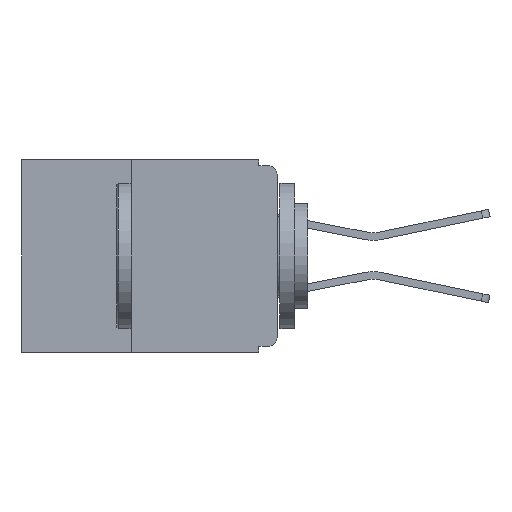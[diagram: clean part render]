
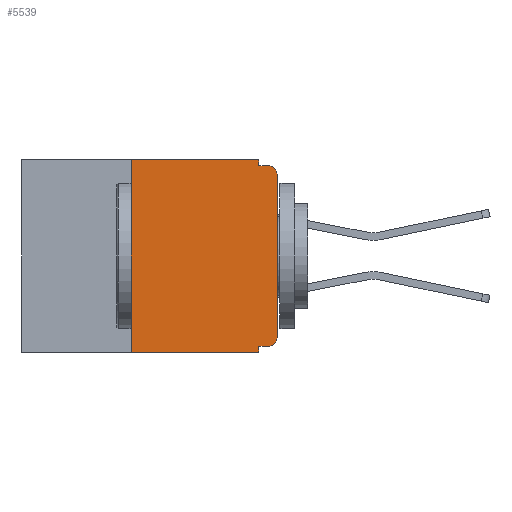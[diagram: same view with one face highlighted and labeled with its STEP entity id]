
A CAD part, left-side view. The second image highlights one B-rep face of the part: STEP entity #5539.
In plain terms, the highlighted planar face has unit normal (-1, 0, 0).
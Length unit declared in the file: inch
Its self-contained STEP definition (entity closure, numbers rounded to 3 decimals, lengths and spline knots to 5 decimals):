
#279 = CARTESIAN_POINT ( 'NONE',  ( 0., 0.031, 0. ) ) ;
#623 = EDGE_CURVE ( 'NONE', #16920, #27429, #1084, .T. ) ;
#801 = DIRECTION ( 'NONE',  ( 0., 0., 1. ) ) ;
#982 = EDGE_CURVE ( 'NONE', #28440, #15134, #9191, .T. ) ;
#1010 = VECTOR ( 'NONE', #801, 39.37008 ) ;
#1084 = CIRCLE ( 'NONE', #10820, 0.015 ) ;
#1388 = CARTESIAN_POINT ( 'NONE',  ( 0., 0.031, -0.32 ) ) ;
#1550 = AXIS2_PLACEMENT_3D ( 'NONE', #21986, #21956, #21898 ) ;
#1650 = VERTEX_POINT ( 'NONE', #13830 ) ;
#1962 = VECTOR ( 'NONE', #7906, 39.37008 ) ;
#1989 = FACE_OUTER_BOUND ( 'NONE', #24034, .T. ) ;
#2897 = CARTESIAN_POINT ( 'NONE',  ( 0., 0., -0.305 ) ) ;
#2940 = PLANE ( 'NONE',  #23125 ) ;
#3177 = VECTOR ( 'NONE', #17419, 39.37008 ) ;
#3666 = EDGE_CURVE ( 'NONE', #4687, #23627, #11005, .T. ) ;
#4248 = CARTESIAN_POINT ( 'NONE',  ( 0., 0.25, -0.33 ) ) ;
#4471 = CARTESIAN_POINT ( 'NONE',  ( 0., 0., -0.025 ) ) ;
#4526 = CARTESIAN_POINT ( 'NONE',  ( 0., 0.437, 0. ) ) ;
#4687 = VERTEX_POINT ( 'NONE', #4471 ) ;
#4823 = ORIENTED_EDGE ( 'NONE', *, *, #15640, .F. ) ;
#5326 = CARTESIAN_POINT ( 'NONE',  ( 0., 0.031, 0. ) ) ;
#5408 = CARTESIAN_POINT ( 'NONE',  ( 0., 0., 0. ) ) ;
#5539 = ADVANCED_FACE ( 'NONE', ( #1989 ), #2940, .F. ) ;
#5545 = LINE ( 'NONE', #25865, #11534 ) ;
#5643 = ORIENTED_EDGE ( 'NONE', *, *, #9518, .F. ) ;
#6651 = ORIENTED_EDGE ( 'NONE', *, *, #14107, .F. ) ;
#6723 = LINE ( 'NONE', #14925, #12059 ) ;
#7178 = CARTESIAN_POINT ( 'NONE',  ( 0., 0.031, -0.33 ) ) ;
#7906 = DIRECTION ( 'NONE',  ( 0., -1., 0. ) ) ;
#7996 = LINE ( 'NONE', #14711, #1962 ) ;
#8221 = EDGE_CURVE ( 'NONE', #16920, #22585, #18970, .T. ) ;
#8771 = VERTEX_POINT ( 'NONE', #7178 ) ;
#8776 = DIRECTION ( 'NONE',  ( 0., 0., 1. ) ) ;
#9191 = LINE ( 'NONE', #4526, #3177 ) ;
#9518 = EDGE_CURVE ( 'NONE', #22585, #8771, #5545, .T. ) ;
#10020 = ORIENTED_EDGE ( 'NONE', *, *, #3666, .T. ) ;
#10310 = DIRECTION ( 'NONE',  ( 0., -1., 0. ) ) ;
#10820 = AXIS2_PLACEMENT_3D ( 'NONE', #20496, #19512, #19413 ) ;
#11005 = CIRCLE ( 'NONE', #1550, 0.015 ) ;
#11534 = VECTOR ( 'NONE', #12198, 39.37008 ) ;
#12059 = VECTOR ( 'NONE', #10310, 39.37008 ) ;
#12084 = CARTESIAN_POINT ( 'NONE',  ( 0., 0.437, 0. ) ) ;
#12198 = DIRECTION ( 'NONE',  ( 0., 0., -1. ) ) ;
#12588 = EDGE_CURVE ( 'NONE', #28463, #8771, #6723, .T. ) ;
#12625 = ORIENTED_EDGE ( 'NONE', *, *, #15866, .F. ) ;
#12907 = VECTOR ( 'NONE', #21074, 39.37008 ) ;
#13012 = VECTOR ( 'NONE', #18476, 39.37008 ) ;
#13095 = LINE ( 'NONE', #5408, #1010 ) ;
#13830 = CARTESIAN_POINT ( 'NONE',  ( 0., 0.031, -0.01 ) ) ;
#14107 = EDGE_CURVE ( 'NONE', #28463, #28440, #19831, .T. ) ;
#14165 = CARTESIAN_POINT ( 'NONE',  ( 0., 0., -0.32 ) ) ;
#14381 = DIRECTION ( 'NONE',  ( 0., 0., -1. ) ) ;
#14711 = CARTESIAN_POINT ( 'NONE',  ( 0., 0., -0.01 ) ) ;
#14925 = CARTESIAN_POINT ( 'NONE',  ( 0., 0.437, -0.33 ) ) ;
#15134 = VERTEX_POINT ( 'NONE', #5326 ) ;
#15640 = EDGE_CURVE ( 'NONE', #15134, #1650, #19074, .T. ) ;
#15866 = EDGE_CURVE ( 'NONE', #1650, #23627, #7996, .T. ) ;
#16920 = VERTEX_POINT ( 'NONE', #25855 ) ;
#17236 = CARTESIAN_POINT ( 'NONE',  ( 0., 0.25, -0.33 ) ) ;
#17419 = DIRECTION ( 'NONE',  ( 0., -1., 0. ) ) ;
#18416 = ORIENTED_EDGE ( 'NONE', *, *, #22007, .T. ) ;
#18476 = DIRECTION ( 'NONE',  ( 0., 0., -1. ) ) ;
#18970 = LINE ( 'NONE', #14165, #12907 ) ;
#19074 = LINE ( 'NONE', #279, #13012 ) ;
#19099 = VECTOR ( 'NONE', #8776, 39.37008 ) ;
#19135 = ORIENTED_EDGE ( 'NONE', *, *, #8221, .F. ) ;
#19413 = DIRECTION ( 'NONE',  ( 0., 0., -1. ) ) ;
#19512 = DIRECTION ( 'NONE',  ( -1., 0., 0. ) ) ;
#19532 = CARTESIAN_POINT ( 'NONE',  ( 0., 0.25, 0. ) ) ;
#19831 = LINE ( 'NONE', #4248, #19099 ) ;
#20496 = CARTESIAN_POINT ( 'NONE',  ( 0., 0.015, -0.305 ) ) ;
#21074 = DIRECTION ( 'NONE',  ( 0., 1., 0. ) ) ;
#21898 = DIRECTION ( 'NONE',  ( 0., 0., -1. ) ) ;
#21956 = DIRECTION ( 'NONE',  ( -1., 0., 0. ) ) ;
#21986 = CARTESIAN_POINT ( 'NONE',  ( 0., 0.015, -0.025 ) ) ;
#22007 = EDGE_CURVE ( 'NONE', #27429, #4687, #13095, .T. ) ;
#22585 = VERTEX_POINT ( 'NONE', #1388 ) ;
#22711 = ORIENTED_EDGE ( 'NONE', *, *, #623, .T. ) ;
#23061 = ORIENTED_EDGE ( 'NONE', *, *, #12588, .T. ) ;
#23125 = AXIS2_PLACEMENT_3D ( 'NONE', #12084, #27974, #14381 ) ;
#23627 = VERTEX_POINT ( 'NONE', #28131 ) ;
#24034 = EDGE_LOOP ( 'NONE', ( #18416, #10020, #12625, #4823, #28618, #6651, #23061, #5643, #19135, #22711 ) ) ;
#25855 = CARTESIAN_POINT ( 'NONE',  ( 0., 0.015, -0.32 ) ) ;
#25865 = CARTESIAN_POINT ( 'NONE',  ( 0., 0.031, -0.33 ) ) ;
#27429 = VERTEX_POINT ( 'NONE', #2897 ) ;
#27974 = DIRECTION ( 'NONE',  ( 1., 0., 0. ) ) ;
#28131 = CARTESIAN_POINT ( 'NONE',  ( 0., 0.015, -0.01 ) ) ;
#28440 = VERTEX_POINT ( 'NONE', #19532 ) ;
#28463 = VERTEX_POINT ( 'NONE', #17236 ) ;
#28618 = ORIENTED_EDGE ( 'NONE', *, *, #982, .F. ) ;
